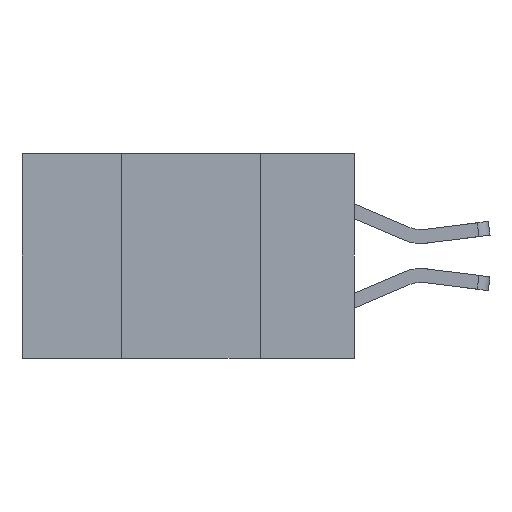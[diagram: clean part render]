
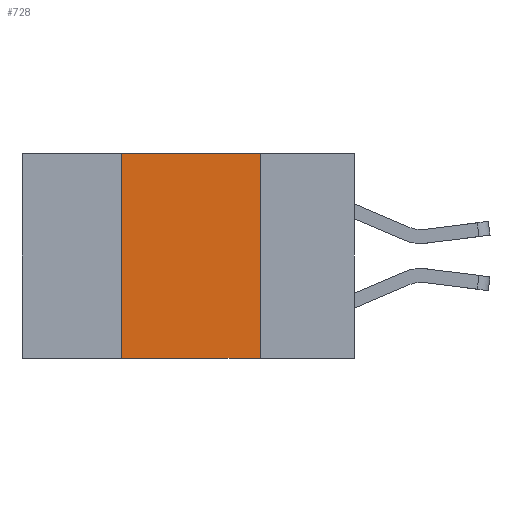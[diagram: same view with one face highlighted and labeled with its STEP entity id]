
A CAD part, left-side view. The second image highlights one B-rep face of the part: STEP entity #728.
In plain terms, the highlighted planar face has unit normal (-1, 0, 0).
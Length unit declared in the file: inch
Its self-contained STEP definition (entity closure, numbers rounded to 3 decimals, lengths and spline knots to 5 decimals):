
#78 = EDGE_CURVE ( 'NONE', #3275, #3109, #4464, .T. ) ;
#728 = ADVANCED_FACE ( 'NONE', ( #9056 ), #4063, .F. ) ;
#905 = CARTESIAN_POINT ( 'NONE',  ( 0., 0.6, 0. ) ) ;
#984 = ORIENTED_EDGE ( 'NONE', *, *, #7844, .T. ) ;
#1074 = CARTESIAN_POINT ( 'NONE',  ( 0., 0.17, 0. ) ) ;
#1222 = VERTEX_POINT ( 'NONE', #10874 ) ;
#1233 = ORIENTED_EDGE ( 'NONE', *, *, #78, .F. ) ;
#1420 = VECTOR ( 'NONE', #1594, 39.37008 ) ;
#1460 = ORIENTED_EDGE ( 'NONE', *, *, #7620, .F. ) ;
#1594 = DIRECTION ( 'NONE',  ( 0., 0., 1. ) ) ;
#1782 = CARTESIAN_POINT ( 'NONE',  ( 0., 0.17, -0.37 ) ) ;
#2028 = VERTEX_POINT ( 'NONE', #8225 ) ;
#2203 = VECTOR ( 'NONE', #7889, 39.37008 ) ;
#2256 = LINE ( 'NONE', #3538, #8717 ) ;
#2388 = CARTESIAN_POINT ( 'NONE',  ( 0., 0.6, 0. ) ) ;
#2686 = DIRECTION ( 'NONE',  ( 0., -1., 0. ) ) ;
#3109 = VERTEX_POINT ( 'NONE', #1782 ) ;
#3132 = ORIENTED_EDGE ( 'NONE', *, *, #4683, .F. ) ;
#3215 = AXIS2_PLACEMENT_3D ( 'NONE', #905, #6835, #5969 ) ;
#3253 = DIRECTION ( 'NONE',  ( 0., -1., 0. ) ) ;
#3275 = VERTEX_POINT ( 'NONE', #1074 ) ;
#3538 = CARTESIAN_POINT ( 'NONE',  ( 0., 0.6, -0.37 ) ) ;
#4063 = PLANE ( 'NONE',  #3215 ) ;
#4396 = VECTOR ( 'NONE', #3253, 39.37008 ) ;
#4464 = LINE ( 'NONE', #7191, #2203 ) ;
#4650 = LINE ( 'NONE', #2388, #4396 ) ;
#4683 = EDGE_CURVE ( 'NONE', #2028, #1222, #10445, .T. ) ;
#5268 = EDGE_LOOP ( 'NONE', ( #1233, #1460, #3132, #984 ) ) ;
#5969 = DIRECTION ( 'NONE',  ( 0., 0., -1. ) ) ;
#6835 = DIRECTION ( 'NONE',  ( 1., 0., 0. ) ) ;
#7191 = CARTESIAN_POINT ( 'NONE',  ( 0., 0.17, 0. ) ) ;
#7450 = CARTESIAN_POINT ( 'NONE',  ( 0., 0.42, 0. ) ) ;
#7620 = EDGE_CURVE ( 'NONE', #1222, #3275, #4650, .T. ) ;
#7844 = EDGE_CURVE ( 'NONE', #2028, #3109, #2256, .T. ) ;
#7889 = DIRECTION ( 'NONE',  ( 0., 0., -1. ) ) ;
#8225 = CARTESIAN_POINT ( 'NONE',  ( 0., 0.42, -0.37 ) ) ;
#8717 = VECTOR ( 'NONE', #2686, 39.37008 ) ;
#9056 = FACE_OUTER_BOUND ( 'NONE', #5268, .T. ) ;
#10445 = LINE ( 'NONE', #7450, #1420 ) ;
#10874 = CARTESIAN_POINT ( 'NONE',  ( 0., 0.42, 0. ) ) ;
